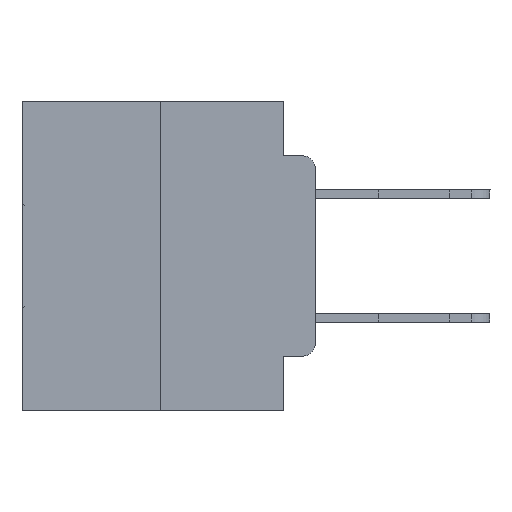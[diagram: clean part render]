
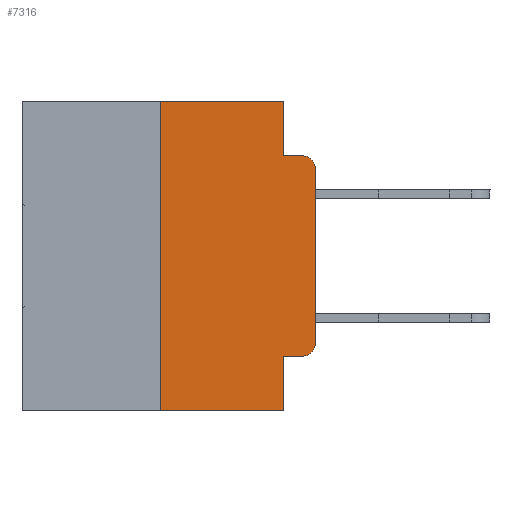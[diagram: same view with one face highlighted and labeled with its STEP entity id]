
A CAD part, left-side view. The second image highlights one B-rep face of the part: STEP entity #7316.
In plain terms, the highlighted planar face has unit normal (-1, 0, 0).
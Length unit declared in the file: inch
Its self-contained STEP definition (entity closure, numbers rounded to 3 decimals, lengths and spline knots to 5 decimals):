
#472 = CARTESIAN_POINT ( 'NONE',  ( 0., 0.02, -0.1085 ) ) ;
#636 = EDGE_CURVE ( 'NONE', #1135, #19623, #23887, .T. ) ;
#669 = ORIENTED_EDGE ( 'NONE', *, *, #18802, .F. ) ;
#934 = DIRECTION ( 'NONE',  ( 0., 0., 1. ) ) ;
#1135 = VERTEX_POINT ( 'NONE', #8034 ) ;
#1774 = DIRECTION ( 'NONE',  ( 0., 0., 1. ) ) ;
#1943 = EDGE_CURVE ( 'NONE', #12814, #21707, #29802, .T. ) ;
#2007 = VECTOR ( 'NONE', #6266, 39.37008 ) ;
#2386 = ORIENTED_EDGE ( 'NONE', *, *, #21882, .T. ) ;
#2471 = ORIENTED_EDGE ( 'NONE', *, *, #29594, .T. ) ;
#2752 = DIRECTION ( 'NONE',  ( 0., 0., -1. ) ) ;
#3031 = DIRECTION ( 'NONE',  ( 0., -1., 0. ) ) ;
#3301 = VERTEX_POINT ( 'NONE', #11653 ) ;
#3506 = AXIS2_PLACEMENT_3D ( 'NONE', #6025, #10886, #3712 ) ;
#3665 = CARTESIAN_POINT ( 'NONE',  ( 0., 0.25, -0.5 ) ) ;
#3712 = DIRECTION ( 'NONE',  ( 0., 0., -1. ) ) ;
#3824 = VERTEX_POINT ( 'NONE', #30593 ) ;
#4370 = LINE ( 'NONE', #25803, #26286 ) ;
#4462 = EDGE_CURVE ( 'NONE', #12814, #19282, #5174, .T. ) ;
#5174 = LINE ( 'NONE', #28970, #30072 ) ;
#5211 = AXIS2_PLACEMENT_3D ( 'NONE', #19988, #15353, #10412 ) ;
#6025 = CARTESIAN_POINT ( 'NONE',  ( 0., 0.02, -0.3915 ) ) ;
#6266 = DIRECTION ( 'NONE',  ( 0., 0., -1. ) ) ;
#7054 = AXIS2_PLACEMENT_3D ( 'NONE', #472, #7525, #2752 ) ;
#7064 = EDGE_LOOP ( 'NONE', ( #23117, #2386, #669, #7167, #28444, #11596, #2471, #25926, #7809, #26465 ) ) ;
#7167 = ORIENTED_EDGE ( 'NONE', *, *, #636, .F. ) ;
#7316 = ADVANCED_FACE ( 'NONE', ( #27229 ), #22514, .F. ) ;
#7525 = DIRECTION ( 'NONE',  ( -1., 0., 0. ) ) ;
#7809 = ORIENTED_EDGE ( 'NONE', *, *, #4462, .T. ) ;
#8034 = CARTESIAN_POINT ( 'NONE',  ( 0., 0.051, 0. ) ) ;
#8523 = CARTESIAN_POINT ( 'NONE',  ( 0., 0., 0. ) ) ;
#9009 = EDGE_CURVE ( 'NONE', #3824, #1135, #18842, .T. ) ;
#9594 = CARTESIAN_POINT ( 'NONE',  ( 0., 0.051, -0.4115 ) ) ;
#10412 = DIRECTION ( 'NONE',  ( 0., 0., -1. ) ) ;
#10886 = DIRECTION ( 'NONE',  ( -1., 0., 0. ) ) ;
#11136 = LINE ( 'NONE', #22326, #25066 ) ;
#11310 = VERTEX_POINT ( 'NONE', #3665 ) ;
#11435 = CARTESIAN_POINT ( 'NONE',  ( 0., 0.051, -0.5 ) ) ;
#11596 = ORIENTED_EDGE ( 'NONE', *, *, #15341, .F. ) ;
#11653 = CARTESIAN_POINT ( 'NONE',  ( 0., 0., -0.3915 ) ) ;
#11999 = LINE ( 'NONE', #29220, #22931 ) ;
#12441 = VECTOR ( 'NONE', #17431, 39.37008 ) ;
#12557 = LINE ( 'NONE', #8523, #24621 ) ;
#12814 = VERTEX_POINT ( 'NONE', #9594 ) ;
#13789 = VERTEX_POINT ( 'NONE', #30605 ) ;
#15082 = VECTOR ( 'NONE', #16304, 39.37008 ) ;
#15341 = EDGE_CURVE ( 'NONE', #11310, #3824, #4370, .T. ) ;
#15353 = DIRECTION ( 'NONE',  ( 1., 0., 0. ) ) ;
#16199 = CARTESIAN_POINT ( 'NONE',  ( 0., 0.051, 0. ) ) ;
#16304 = DIRECTION ( 'NONE',  ( 0., 0., -1. ) ) ;
#17431 = DIRECTION ( 'NONE',  ( 0., -1., 0. ) ) ;
#18107 = EDGE_CURVE ( 'NONE', #19282, #3301, #24139, .T. ) ;
#18802 = EDGE_CURVE ( 'NONE', #19623, #22696, #11999, .T. ) ;
#18842 = LINE ( 'NONE', #22907, #12441 ) ;
#19282 = VERTEX_POINT ( 'NONE', #23516 ) ;
#19580 = CARTESIAN_POINT ( 'NONE',  ( 0., 0.02, -0.0885 ) ) ;
#19623 = VERTEX_POINT ( 'NONE', #27710 ) ;
#19917 = DIRECTION ( 'NONE',  ( 0., -1., 0. ) ) ;
#19988 = CARTESIAN_POINT ( 'NONE',  ( 0., 0.473, 0. ) ) ;
#20093 = DIRECTION ( 'NONE',  ( 0., -1., 0. ) ) ;
#21707 = VERTEX_POINT ( 'NONE', #11435 ) ;
#21882 = EDGE_CURVE ( 'NONE', #13789, #22696, #22717, .T. ) ;
#22326 = CARTESIAN_POINT ( 'NONE',  ( 0., 0.473, -0.5 ) ) ;
#22514 = PLANE ( 'NONE',  #5211 ) ;
#22696 = VERTEX_POINT ( 'NONE', #19580 ) ;
#22717 = CIRCLE ( 'NONE', #7054, 0.02 ) ;
#22907 = CARTESIAN_POINT ( 'NONE',  ( 0., 0.473, 0. ) ) ;
#22931 = VECTOR ( 'NONE', #19917, 39.37008 ) ;
#23117 = ORIENTED_EDGE ( 'NONE', *, *, #24665, .T. ) ;
#23516 = CARTESIAN_POINT ( 'NONE',  ( 0., 0.02, -0.4115 ) ) ;
#23887 = LINE ( 'NONE', #30406, #2007 ) ;
#24139 = CIRCLE ( 'NONE', #3506, 0.02 ) ;
#24621 = VECTOR ( 'NONE', #934, 39.37008 ) ;
#24665 = EDGE_CURVE ( 'NONE', #3301, #13789, #12557, .T. ) ;
#25066 = VECTOR ( 'NONE', #20093, 39.37008 ) ;
#25803 = CARTESIAN_POINT ( 'NONE',  ( 0., 0.25, 0. ) ) ;
#25926 = ORIENTED_EDGE ( 'NONE', *, *, #1943, .F. ) ;
#26286 = VECTOR ( 'NONE', #1774, 39.37008 ) ;
#26465 = ORIENTED_EDGE ( 'NONE', *, *, #18107, .T. ) ;
#27229 = FACE_OUTER_BOUND ( 'NONE', #7064, .T. ) ;
#27710 = CARTESIAN_POINT ( 'NONE',  ( 0., 0.051, -0.0885 ) ) ;
#28444 = ORIENTED_EDGE ( 'NONE', *, *, #9009, .F. ) ;
#28970 = CARTESIAN_POINT ( 'NONE',  ( 0., 0.051, -0.4115 ) ) ;
#29220 = CARTESIAN_POINT ( 'NONE',  ( 0., 0.051, -0.0885 ) ) ;
#29594 = EDGE_CURVE ( 'NONE', #11310, #21707, #11136, .T. ) ;
#29802 = LINE ( 'NONE', #16199, #15082 ) ;
#30072 = VECTOR ( 'NONE', #3031, 39.37008 ) ;
#30406 = CARTESIAN_POINT ( 'NONE',  ( 0., 0.051, 0. ) ) ;
#30593 = CARTESIAN_POINT ( 'NONE',  ( 0., 0.25, 0. ) ) ;
#30605 = CARTESIAN_POINT ( 'NONE',  ( 0., 0., -0.1085 ) ) ;
